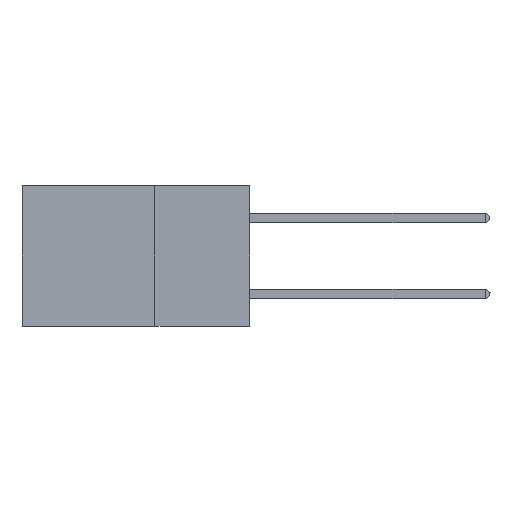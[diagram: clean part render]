
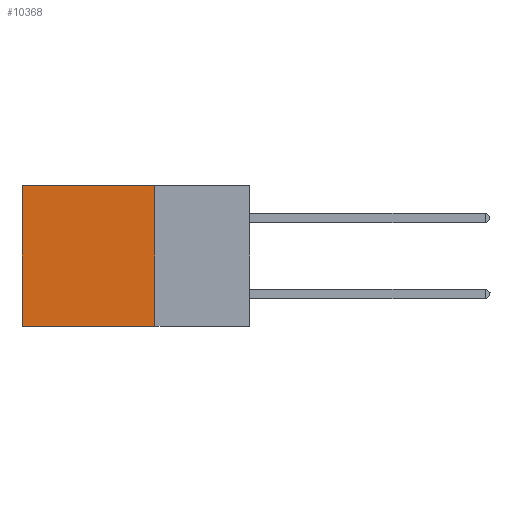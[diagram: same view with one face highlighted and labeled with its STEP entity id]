
A CAD part, left-side view. The second image highlights one B-rep face of the part: STEP entity #10368.
In plain terms, the highlighted planar face has unit normal (-1, 0, 0).
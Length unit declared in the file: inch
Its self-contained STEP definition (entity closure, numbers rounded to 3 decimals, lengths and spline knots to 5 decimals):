
#684 = ORIENTED_EDGE ( 'NONE', *, *, #4030, .F. ) ;
#1082 = VECTOR ( 'NONE', #7837, 39.37008 ) ;
#1147 = CARTESIAN_POINT ( 'NONE',  ( 0.2875, 0.25, 0. ) ) ;
#1429 = VECTOR ( 'NONE', #4294, 39.37008 ) ;
#2382 = CARTESIAN_POINT ( 'NONE',  ( 0.2875, 0.6, 0. ) ) ;
#2649 = VERTEX_POINT ( 'NONE', #17876 ) ;
#2898 = DIRECTION ( 'NONE',  ( 0., 0., -1. ) ) ;
#2922 = DIRECTION ( 'NONE',  ( 0., 0., -1. ) ) ;
#3327 = ORIENTED_EDGE ( 'NONE', *, *, #12087, .F. ) ;
#4030 = EDGE_CURVE ( 'NONE', #11736, #7849, #17942, .T. ) ;
#4291 = ORIENTED_EDGE ( 'NONE', *, *, #15370, .T. ) ;
#4294 = DIRECTION ( 'NONE',  ( 0., 1., 0. ) ) ;
#4539 = ORIENTED_EDGE ( 'NONE', *, *, #20238, .T. ) ;
#4567 = CARTESIAN_POINT ( 'NONE',  ( 0.2875, 0.6, 0. ) ) ;
#5495 = AXIS2_PLACEMENT_3D ( 'NONE', #12896, #14238, #2898 ) ;
#6096 = CARTESIAN_POINT ( 'NONE',  ( 0.2875, 0.25, -0.37 ) ) ;
#6736 = VECTOR ( 'NONE', #21542, 39.37008 ) ;
#7837 = DIRECTION ( 'NONE',  ( 0., 0., -1. ) ) ;
#7849 = VERTEX_POINT ( 'NONE', #20393 ) ;
#8264 = VECTOR ( 'NONE', #2922, 39.37008 ) ;
#10368 = ADVANCED_FACE ( 'NONE', ( #14126 ), #14462, .F. ) ;
#11736 = VERTEX_POINT ( 'NONE', #6096 ) ;
#12087 = EDGE_CURVE ( 'NONE', #2649, #11736, #12775, .T. ) ;
#12775 = LINE ( 'NONE', #1147, #1082 ) ;
#12896 = CARTESIAN_POINT ( 'NONE',  ( 0.2875, 0.25, 0. ) ) ;
#12918 = LINE ( 'NONE', #4567, #8264 ) ;
#12933 = EDGE_LOOP ( 'NONE', ( #4539, #684, #3327, #4291 ) ) ;
#14126 = FACE_OUTER_BOUND ( 'NONE', #12933, .T. ) ;
#14238 = DIRECTION ( 'NONE',  ( 1., 0., 0. ) ) ;
#14422 = CARTESIAN_POINT ( 'NONE',  ( 0.2875, 0.25, -0.37 ) ) ;
#14462 = PLANE ( 'NONE',  #5495 ) ;
#15046 = LINE ( 'NONE', #18250, #6736 ) ;
#15370 = EDGE_CURVE ( 'NONE', #2649, #20027, #15046, .T. ) ;
#17876 = CARTESIAN_POINT ( 'NONE',  ( 0.2875, 0.25, 0. ) ) ;
#17942 = LINE ( 'NONE', #14422, #1429 ) ;
#18250 = CARTESIAN_POINT ( 'NONE',  ( 0.2875, 0.25, 0. ) ) ;
#20027 = VERTEX_POINT ( 'NONE', #2382 ) ;
#20238 = EDGE_CURVE ( 'NONE', #20027, #7849, #12918, .T. ) ;
#20393 = CARTESIAN_POINT ( 'NONE',  ( 0.2875, 0.6, -0.37 ) ) ;
#21542 = DIRECTION ( 'NONE',  ( 0., 1., 0. ) ) ;
